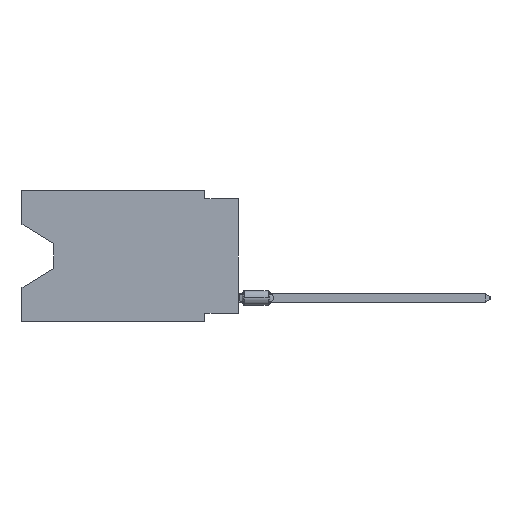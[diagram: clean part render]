
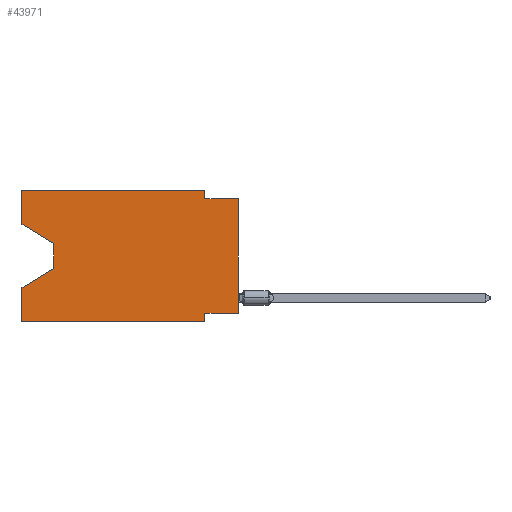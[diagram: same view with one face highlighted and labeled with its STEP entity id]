
A CAD part, left-side view. The second image highlights one B-rep face of the part: STEP entity #43971.
In plain terms, the highlighted planar face has unit normal (-1, 0, 0).
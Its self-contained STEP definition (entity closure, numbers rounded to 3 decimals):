
#404 = CARTESIAN_POINT ( 'NONE',  ( 0., 0., -0.635 ) ) ;
#1208 = EDGE_CURVE ( 'NONE', #70518, #49238, #9900, .T. ) ;
#1491 = CARTESIAN_POINT ( 'NONE',  ( 0., 16.383, 0. ) ) ;
#2802 = CARTESIAN_POINT ( 'NONE',  ( 0., 2.54, 0. ) ) ;
#4719 = CARTESIAN_POINT ( 'NONE',  ( 0., 2.54, -9.906 ) ) ;
#6007 = VERTEX_POINT ( 'NONE', #12668 ) ;
#6267 = VERTEX_POINT ( 'NONE', #2802 ) ;
#8502 = LINE ( 'NONE', #64291, #62434 ) ;
#9403 = CARTESIAN_POINT ( 'NONE',  ( 0., 16.383, -9.906 ) ) ;
#9686 = DIRECTION ( 'NONE',  ( 0., 0., 1. ) ) ;
#9900 = LINE ( 'NONE', #59432, #23191 ) ;
#10032 = VERTEX_POINT ( 'NONE', #26178 ) ;
#10205 = LINE ( 'NONE', #20911, #20358 ) ;
#10878 = EDGE_LOOP ( 'NONE', ( #56520, #45329, #12650, #33448, #47352, #14511, #61225, #19386, #46910, #20810, #62692, #13699 ) ) ;
#12561 = VERTEX_POINT ( 'NONE', #40722 ) ;
#12650 = ORIENTED_EDGE ( 'NONE', *, *, #55510, .T. ) ;
#12668 = CARTESIAN_POINT ( 'NONE',  ( 0., 16.383, -7.36 ) ) ;
#13415 = CARTESIAN_POINT ( 'NONE',  ( 0., 2.54, -9.906 ) ) ;
#13481 = CARTESIAN_POINT ( 'NONE',  ( 0., 0., 0. ) ) ;
#13699 = ORIENTED_EDGE ( 'NONE', *, *, #47770, .F. ) ;
#13962 = VERTEX_POINT ( 'NONE', #4719 ) ;
#14511 = ORIENTED_EDGE ( 'NONE', *, *, #58078, .F. ) ;
#14863 = LINE ( 'NONE', #47757, #62342 ) ;
#15411 = DIRECTION ( 'NONE',  ( 0., 0., -1. ) ) ;
#16828 = CARTESIAN_POINT ( 'NONE',  ( 0., 13.97, -4.013 ) ) ;
#16941 = CARTESIAN_POINT ( 'NONE',  ( 0., 2.54, -9.271 ) ) ;
#19386 = ORIENTED_EDGE ( 'NONE', *, *, #23025, .T. ) ;
#19855 = EDGE_CURVE ( 'NONE', #32700, #70518, #50770, .T. ) ;
#20358 = VECTOR ( 'NONE', #26442, 1000. ) ;
#20810 = ORIENTED_EDGE ( 'NONE', *, *, #47048, .F. ) ;
#20911 = CARTESIAN_POINT ( 'NONE',  ( 0., 0., -9.271 ) ) ;
#21449 = DIRECTION ( 'NONE',  ( 0., 0.855, -0.519 ) ) ;
#23025 = EDGE_CURVE ( 'NONE', #71819, #39090, #29759, .T. ) ;
#23191 = VECTOR ( 'NONE', #60531, 1000. ) ;
#23844 = VECTOR ( 'NONE', #53216, 1000. ) ;
#25406 = VERTEX_POINT ( 'NONE', #16941 ) ;
#25758 = VECTOR ( 'NONE', #32274, 1000. ) ;
#26178 = CARTESIAN_POINT ( 'NONE',  ( 0., 16.383, 0. ) ) ;
#26442 = DIRECTION ( 'NONE',  ( 0., 1., 0. ) ) ;
#26482 = CARTESIAN_POINT ( 'NONE',  ( 0., 16.383, 0. ) ) ;
#29688 = CARTESIAN_POINT ( 'NONE',  ( 0., 16.383, -2.546 ) ) ;
#29759 = LINE ( 'NONE', #13481, #36130 ) ;
#30250 = VERTEX_POINT ( 'NONE', #57213 ) ;
#30474 = CARTESIAN_POINT ( 'NONE',  ( 0., 2.54, 0. ) ) ;
#31187 = LINE ( 'NONE', #30474, #39662 ) ;
#32274 = DIRECTION ( 'NONE',  ( 0., -1., 0. ) ) ;
#32686 = LINE ( 'NONE', #37503, #44095 ) ;
#32700 = VERTEX_POINT ( 'NONE', #39871 ) ;
#33448 = ORIENTED_EDGE ( 'NONE', *, *, #35534, .F. ) ;
#34889 = LINE ( 'NONE', #13415, #64273 ) ;
#35248 = DIRECTION ( 'NONE',  ( 0., 0., -1. ) ) ;
#35534 = EDGE_CURVE ( 'NONE', #30250, #6007, #14863, .T. ) ;
#36130 = VECTOR ( 'NONE', #63771, 1000. ) ;
#36989 = VECTOR ( 'NONE', #21449, 1000. ) ;
#37437 = EDGE_CURVE ( 'NONE', #30250, #13962, #66297, .T. ) ;
#37503 = CARTESIAN_POINT ( 'NONE',  ( 0., 16.383, 0. ) ) ;
#37950 = DIRECTION ( 'NONE',  ( 1., 0., 0. ) ) ;
#38091 = EDGE_CURVE ( 'NONE', #12561, #39090, #8502, .T. ) ;
#39090 = VERTEX_POINT ( 'NONE', #404 ) ;
#39662 = VECTOR ( 'NONE', #47835, 1000. ) ;
#39871 = CARTESIAN_POINT ( 'NONE',  ( 0., 16.383, -2.546 ) ) ;
#40722 = CARTESIAN_POINT ( 'NONE',  ( 0., 2.54, -0.635 ) ) ;
#43971 = ADVANCED_FACE ( 'NONE', ( #65684 ), #60498, .F. ) ;
#44095 = VECTOR ( 'NONE', #72587, 1000. ) ;
#44184 = CARTESIAN_POINT ( 'NONE',  ( 0., 0., -9.271 ) ) ;
#44432 = EDGE_CURVE ( 'NONE', #10032, #6267, #32686, .T. ) ;
#45329 = ORIENTED_EDGE ( 'NONE', *, *, #1208, .T. ) ;
#46910 = ORIENTED_EDGE ( 'NONE', *, *, #38091, .F. ) ;
#47048 = EDGE_CURVE ( 'NONE', #6267, #12561, #31187, .T. ) ;
#47352 = ORIENTED_EDGE ( 'NONE', *, *, #37437, .T. ) ;
#47757 = CARTESIAN_POINT ( 'NONE',  ( 0., 16.383, 0. ) ) ;
#47770 = EDGE_CURVE ( 'NONE', #32700, #10032, #63202, .T. ) ;
#47835 = DIRECTION ( 'NONE',  ( 0., 0., -1. ) ) ;
#49238 = VERTEX_POINT ( 'NONE', #71818 ) ;
#49896 = LINE ( 'NONE', #50633, #36989 ) ;
#50633 = CARTESIAN_POINT ( 'NONE',  ( 0., 13.97, -5.893 ) ) ;
#50770 = LINE ( 'NONE', #29688, #70140 ) ;
#52228 = DIRECTION ( 'NONE',  ( 0., -0.855, -0.519 ) ) ;
#53216 = DIRECTION ( 'NONE',  ( 0., 0., 1. ) ) ;
#54648 = AXIS2_PLACEMENT_3D ( 'NONE', #26482, #37950, #15411 ) ;
#55510 = EDGE_CURVE ( 'NONE', #49238, #6007, #49896, .T. ) ;
#56520 = ORIENTED_EDGE ( 'NONE', *, *, #19855, .T. ) ;
#57213 = CARTESIAN_POINT ( 'NONE',  ( 0., 16.383, -9.906 ) ) ;
#58078 = EDGE_CURVE ( 'NONE', #25406, #13962, #34889, .T. ) ;
#59432 = CARTESIAN_POINT ( 'NONE',  ( 0., 13.97, -4.013 ) ) ;
#60498 = PLANE ( 'NONE',  #54648 ) ;
#60531 = DIRECTION ( 'NONE',  ( 0., 0., -1. ) ) ;
#61225 = ORIENTED_EDGE ( 'NONE', *, *, #71879, .F. ) ;
#62342 = VECTOR ( 'NONE', #9686, 1000. ) ;
#62434 = VECTOR ( 'NONE', #63569, 1000. ) ;
#62692 = ORIENTED_EDGE ( 'NONE', *, *, #44432, .F. ) ;
#63202 = LINE ( 'NONE', #1491, #23844 ) ;
#63569 = DIRECTION ( 'NONE',  ( 0., -1., 0. ) ) ;
#63771 = DIRECTION ( 'NONE',  ( 0., 0., 1. ) ) ;
#64273 = VECTOR ( 'NONE', #35248, 1000. ) ;
#64291 = CARTESIAN_POINT ( 'NONE',  ( 0., 0., -0.635 ) ) ;
#65684 = FACE_OUTER_BOUND ( 'NONE', #10878, .T. ) ;
#66297 = LINE ( 'NONE', #9403, #25758 ) ;
#70140 = VECTOR ( 'NONE', #52228, 1000. ) ;
#70518 = VERTEX_POINT ( 'NONE', #16828 ) ;
#71818 = CARTESIAN_POINT ( 'NONE',  ( 0., 13.97, -5.893 ) ) ;
#71819 = VERTEX_POINT ( 'NONE', #44184 ) ;
#71879 = EDGE_CURVE ( 'NONE', #71819, #25406, #10205, .T. ) ;
#72587 = DIRECTION ( 'NONE',  ( 0., -1., 0. ) ) ;
